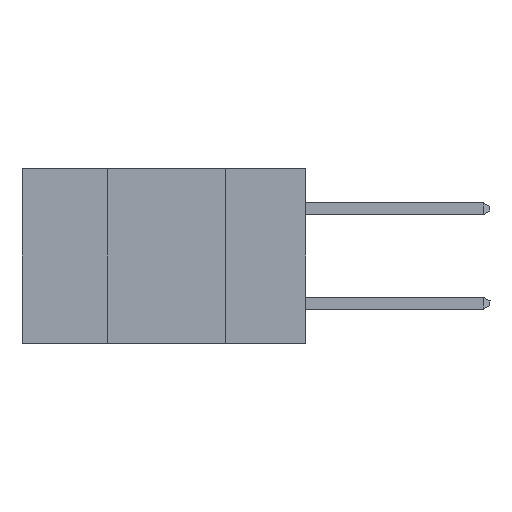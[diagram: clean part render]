
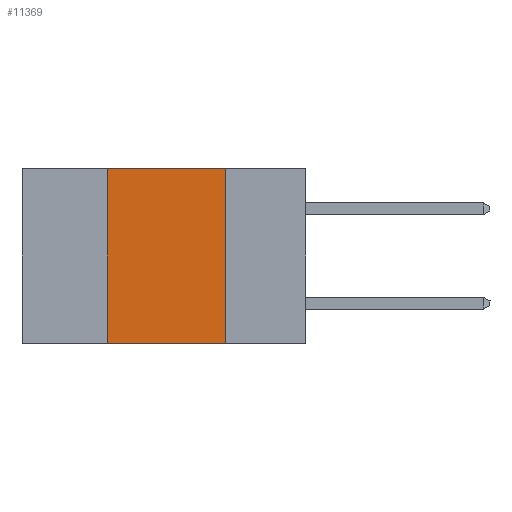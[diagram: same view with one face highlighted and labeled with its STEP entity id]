
A CAD part, left-side view. The second image highlights one B-rep face of the part: STEP entity #11369.
In plain terms, the highlighted planar face has unit normal (-1, 0, 0).
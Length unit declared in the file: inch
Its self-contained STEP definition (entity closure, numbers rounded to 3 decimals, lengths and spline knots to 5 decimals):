
#31 = VERTEX_POINT ( 'NONE', #12268 ) ;
#77 = AXIS2_PLACEMENT_3D ( 'NONE', #11557, #2796, #2919 ) ;
#103 = EDGE_LOOP ( 'NONE', ( #12200, #7450, #743, #1092 ) ) ;
#430 = CARTESIAN_POINT ( 'NONE',  ( 0., 0.17, 0. ) ) ;
#743 = ORIENTED_EDGE ( 'NONE', *, *, #11370, .F. ) ;
#1092 = ORIENTED_EDGE ( 'NONE', *, *, #10654, .T. ) ;
#2255 = FACE_OUTER_BOUND ( 'NONE', #103, .T. ) ;
#2796 = DIRECTION ( 'NONE',  ( 1., 0., 0. ) ) ;
#2877 = PLANE ( 'NONE',  #77 ) ;
#2919 = DIRECTION ( 'NONE',  ( 0., 0., -1. ) ) ;
#3064 = VECTOR ( 'NONE', #8006, 39.37008 ) ;
#3139 = CARTESIAN_POINT ( 'NONE',  ( 0., 0.6, 0. ) ) ;
#3612 = LINE ( 'NONE', #3139, #4630 ) ;
#4301 = EDGE_CURVE ( 'NONE', #8945, #31, #5112, .T. ) ;
#4630 = VECTOR ( 'NONE', #9589, 39.37008 ) ;
#5112 = LINE ( 'NONE', #430, #3064 ) ;
#5123 = CARTESIAN_POINT ( 'NONE',  ( 0., 0.42, 0. ) ) ;
#7406 = VERTEX_POINT ( 'NONE', #8368 ) ;
#7450 = ORIENTED_EDGE ( 'NONE', *, *, #11568, .F. ) ;
#8006 = DIRECTION ( 'NONE',  ( 0., 0., -1. ) ) ;
#8368 = CARTESIAN_POINT ( 'NONE',  ( 0., 0.42, 0. ) ) ;
#8945 = VERTEX_POINT ( 'NONE', #11328 ) ;
#9589 = DIRECTION ( 'NONE',  ( 0., -1., 0. ) ) ;
#9886 = CARTESIAN_POINT ( 'NONE',  ( 0., 0.6, -0.37 ) ) ;
#10574 = LINE ( 'NONE', #9886, #11593 ) ;
#10654 = EDGE_CURVE ( 'NONE', #11448, #31, #10574, .T. ) ;
#11328 = CARTESIAN_POINT ( 'NONE',  ( 0., 0.17, 0. ) ) ;
#11369 = ADVANCED_FACE ( 'NONE', ( #2255 ), #2877, .F. ) ;
#11370 = EDGE_CURVE ( 'NONE', #11448, #7406, #12918, .T. ) ;
#11448 = VERTEX_POINT ( 'NONE', #13225 ) ;
#11557 = CARTESIAN_POINT ( 'NONE',  ( 0., 0.6, 0. ) ) ;
#11568 = EDGE_CURVE ( 'NONE', #7406, #8945, #3612, .T. ) ;
#11593 = VECTOR ( 'NONE', #12131, 39.37008 ) ;
#12131 = DIRECTION ( 'NONE',  ( 0., -1., 0. ) ) ;
#12200 = ORIENTED_EDGE ( 'NONE', *, *, #4301, .F. ) ;
#12268 = CARTESIAN_POINT ( 'NONE',  ( 0., 0.17, -0.37 ) ) ;
#12443 = VECTOR ( 'NONE', #13716, 39.37008 ) ;
#12918 = LINE ( 'NONE', #5123, #12443 ) ;
#13225 = CARTESIAN_POINT ( 'NONE',  ( 0., 0.42, -0.37 ) ) ;
#13716 = DIRECTION ( 'NONE',  ( 0., 0., 1. ) ) ;
